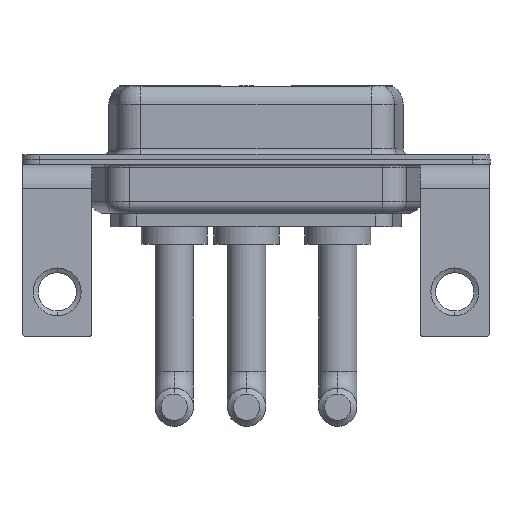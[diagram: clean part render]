
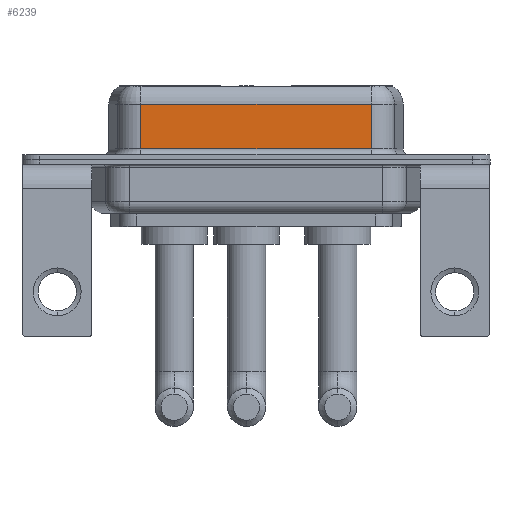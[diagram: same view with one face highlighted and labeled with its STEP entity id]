
A CAD part, front view. The second image highlights one B-rep face of the part: STEP entity #6239.
In plain terms, the highlighted planar face has unit normal (0, -1, 0).
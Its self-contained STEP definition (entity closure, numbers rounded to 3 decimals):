
#158 = VERTEX_POINT ( 'NONE', #3717 ) ;
#525 = CARTESIAN_POINT ( 'NONE',  ( 7.013, -3.95, 4.65 ) ) ;
#706 = EDGE_CURVE ( 'NONE', #4787, #3939, #1723, .T. ) ;
#919 = CARTESIAN_POINT ( 'NONE',  ( 26.287, -3.95, 6.4 ) ) ;
#1358 = LINE ( 'NONE', #5848, #11416 ) ;
#1709 = CARTESIAN_POINT ( 'NONE',  ( 26.287, -3.95, 0.9 ) ) ;
#1723 = LINE ( 'NONE', #7310, #3474 ) ;
#1816 = VECTOR ( 'NONE', #12360, 1000. ) ;
#1851 = EDGE_CURVE ( 'NONE', #8365, #158, #14390, .T. ) ;
#2028 = FACE_OUTER_BOUND ( 'NONE', #14141, .T. ) ;
#2236 = DIRECTION ( 'NONE',  ( 0., 1., 0. ) ) ;
#3340 = DIRECTION ( 'NONE',  ( 0., 0., -1. ) ) ;
#3474 = VECTOR ( 'NONE', #14145, 1000. ) ;
#3717 = CARTESIAN_POINT ( 'NONE',  ( 7.013, -3.95, 0.9 ) ) ;
#3939 = VERTEX_POINT ( 'NONE', #1709 ) ;
#4787 = VERTEX_POINT ( 'NONE', #5249 ) ;
#5249 = CARTESIAN_POINT ( 'NONE',  ( 26.287, -3.95, 4.65 ) ) ;
#5404 = DIRECTION ( 'NONE',  ( 0., 0., 1. ) ) ;
#5529 = CARTESIAN_POINT ( 'NONE',  ( 26.287, -3.95, 0.9 ) ) ;
#5848 = CARTESIAN_POINT ( 'NONE',  ( 26.287, -3.95, 4.65 ) ) ;
#6239 = ADVANCED_FACE ( 'NONE', ( #2028 ), #11232, .F. ) ;
#6502 = ORIENTED_EDGE ( 'NONE', *, *, #11507, .T. ) ;
#7045 = ORIENTED_EDGE ( 'NONE', *, *, #1851, .T. ) ;
#7310 = CARTESIAN_POINT ( 'NONE',  ( 26.287, -3.95, 6.4 ) ) ;
#7925 = ORIENTED_EDGE ( 'NONE', *, *, #706, .F. ) ;
#8365 = VERTEX_POINT ( 'NONE', #525 ) ;
#9844 = CARTESIAN_POINT ( 'NONE',  ( 7.013, -3.95, 6.4 ) ) ;
#10318 = LINE ( 'NONE', #5529, #1816 ) ;
#11232 = PLANE ( 'NONE',  #13658 ) ;
#11294 = VECTOR ( 'NONE', #3340, 1000. ) ;
#11416 = VECTOR ( 'NONE', #13564, 1000. ) ;
#11507 = EDGE_CURVE ( 'NONE', #4787, #8365, #1358, .T. ) ;
#12360 = DIRECTION ( 'NONE',  ( 1., 0., 0. ) ) ;
#13134 = EDGE_CURVE ( 'NONE', #158, #3939, #10318, .T. ) ;
#13362 = ORIENTED_EDGE ( 'NONE', *, *, #13134, .T. ) ;
#13564 = DIRECTION ( 'NONE',  ( -1., 0., 0. ) ) ;
#13658 = AXIS2_PLACEMENT_3D ( 'NONE', #919, #2236, #5404 ) ;
#14141 = EDGE_LOOP ( 'NONE', ( #7925, #6502, #7045, #13362 ) ) ;
#14145 = DIRECTION ( 'NONE',  ( 0., 0., -1. ) ) ;
#14390 = LINE ( 'NONE', #9844, #11294 ) ;
